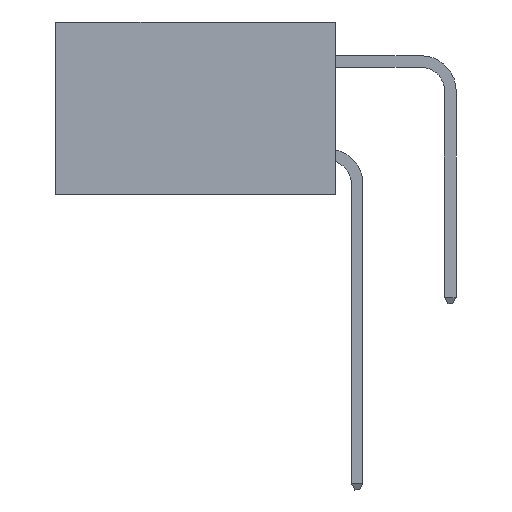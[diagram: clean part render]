
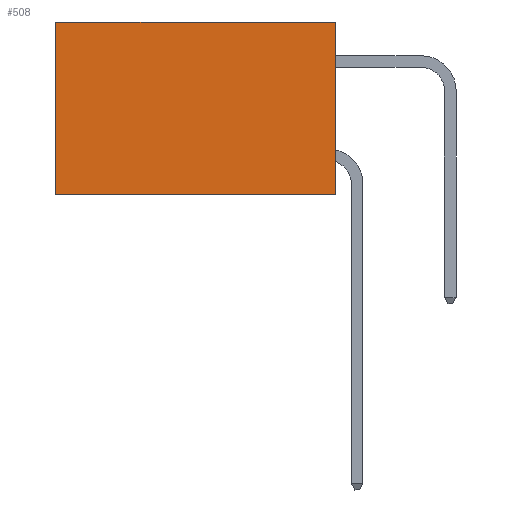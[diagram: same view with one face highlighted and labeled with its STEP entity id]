
A CAD part, left-side view. The second image highlights one B-rep face of the part: STEP entity #508.
In plain terms, the highlighted planar face has unit normal (-1, 0, 0).
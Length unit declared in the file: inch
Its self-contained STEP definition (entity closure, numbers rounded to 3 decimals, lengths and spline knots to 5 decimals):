
#225 = VERTEX_POINT ( 'NONE', #9705 ) ;
#508 = ADVANCED_FACE ( 'NONE', ( #2943 ), #6601, .F. ) ;
#797 = VECTOR ( 'NONE', #5851, 39.37008 ) ;
#962 = CARTESIAN_POINT ( 'NONE',  ( 0.2875, 0.6, 0. ) ) ;
#1487 = EDGE_CURVE ( 'NONE', #4021, #225, #4123, .T. ) ;
#1495 = EDGE_LOOP ( 'NONE', ( #9879, #5655, #5462, #9422 ) ) ;
#1674 = CARTESIAN_POINT ( 'NONE',  ( 0.2875, 0., 0. ) ) ;
#1989 = DIRECTION ( 'NONE',  ( 0., 1., 0. ) ) ;
#2869 = EDGE_CURVE ( 'NONE', #4620, #5946, #6077, .T. ) ;
#2943 = FACE_OUTER_BOUND ( 'NONE', #1495, .T. ) ;
#3283 = DIRECTION ( 'NONE',  ( 1., 0., 0. ) ) ;
#3926 = EDGE_CURVE ( 'NONE', #4021, #4620, #4338, .T. ) ;
#4008 = DIRECTION ( 'NONE',  ( 0., 0., -1. ) ) ;
#4021 = VERTEX_POINT ( 'NONE', #8368 ) ;
#4123 = LINE ( 'NONE', #1674, #797 ) ;
#4338 = LINE ( 'NONE', #6204, #7240 ) ;
#4620 = VERTEX_POINT ( 'NONE', #962 ) ;
#4972 = AXIS2_PLACEMENT_3D ( 'NONE', #10028, #3283, #4008 ) ;
#5043 = VECTOR ( 'NONE', #7790, 39.37008 ) ;
#5462 = ORIENTED_EDGE ( 'NONE', *, *, #1487, .F. ) ;
#5555 = DIRECTION ( 'NONE',  ( 0., 1., 0. ) ) ;
#5655 = ORIENTED_EDGE ( 'NONE', *, *, #6595, .F. ) ;
#5851 = DIRECTION ( 'NONE',  ( 0., 0., -1. ) ) ;
#5946 = VERTEX_POINT ( 'NONE', #9570 ) ;
#6077 = LINE ( 'NONE', #10321, #5043 ) ;
#6204 = CARTESIAN_POINT ( 'NONE',  ( 0.2875, 0., 0. ) ) ;
#6595 = EDGE_CURVE ( 'NONE', #225, #5946, #6814, .T. ) ;
#6601 = PLANE ( 'NONE',  #4972 ) ;
#6814 = LINE ( 'NONE', #8163, #8780 ) ;
#7240 = VECTOR ( 'NONE', #1989, 39.37008 ) ;
#7790 = DIRECTION ( 'NONE',  ( 0., 0., -1. ) ) ;
#8163 = CARTESIAN_POINT ( 'NONE',  ( 0.2875, 0., -0.37 ) ) ;
#8368 = CARTESIAN_POINT ( 'NONE',  ( 0.2875, 0., 0. ) ) ;
#8780 = VECTOR ( 'NONE', #5555, 39.37008 ) ;
#9422 = ORIENTED_EDGE ( 'NONE', *, *, #3926, .T. ) ;
#9570 = CARTESIAN_POINT ( 'NONE',  ( 0.2875, 0.6, -0.37 ) ) ;
#9705 = CARTESIAN_POINT ( 'NONE',  ( 0.2875, 0., -0.37 ) ) ;
#9879 = ORIENTED_EDGE ( 'NONE', *, *, #2869, .T. ) ;
#10028 = CARTESIAN_POINT ( 'NONE',  ( 0.2875, 0., 0. ) ) ;
#10321 = CARTESIAN_POINT ( 'NONE',  ( 0.2875, 0.6, 0. ) ) ;
